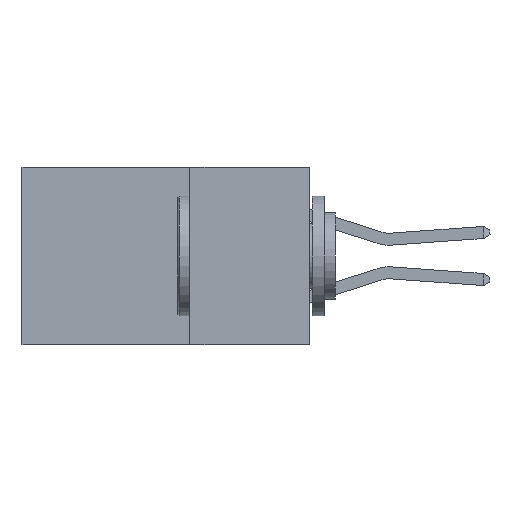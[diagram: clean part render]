
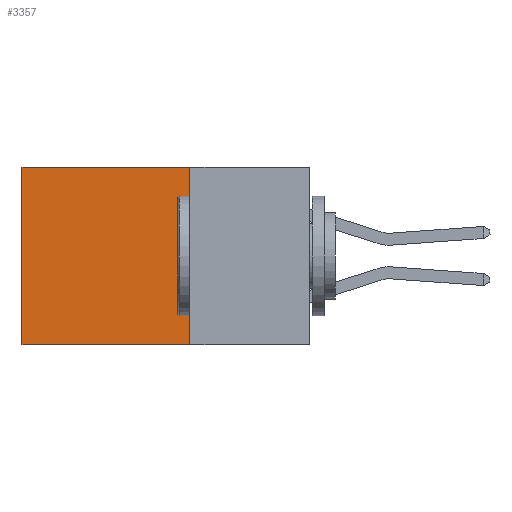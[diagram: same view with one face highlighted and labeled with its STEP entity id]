
A CAD part, left-side view. The second image highlights one B-rep face of the part: STEP entity #3357.
In plain terms, the highlighted planar face has unit normal (-1, 0, 0).
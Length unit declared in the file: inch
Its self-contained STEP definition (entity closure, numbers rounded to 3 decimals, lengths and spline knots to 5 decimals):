
#457 = CARTESIAN_POINT ( 'NONE',  ( 0.298, 0.6, 0. ) ) ;
#503 = CARTESIAN_POINT ( 'NONE',  ( 0.298, 0.25, 0. ) ) ;
#523 = DIRECTION ( 'NONE',  ( 0., 0., -1. ) ) ;
#626 = VECTOR ( 'NONE', #11595, 39.37008 ) ;
#689 = DIRECTION ( 'NONE',  ( 1., 0., 0. ) ) ;
#766 = DIRECTION ( 'NONE',  ( 0., 1., 0. ) ) ;
#1103 = FACE_OUTER_BOUND ( 'NONE', #9966, .T. ) ;
#1236 = LINE ( 'NONE', #457, #626 ) ;
#1303 = CARTESIAN_POINT ( 'NONE',  ( 0.298, 0.25, 0. ) ) ;
#1357 = VECTOR ( 'NONE', #10950, 39.37008 ) ;
#1670 = VERTEX_POINT ( 'NONE', #6899 ) ;
#2214 = ORIENTED_EDGE ( 'NONE', *, *, #8538, .F. ) ;
#2827 = ORIENTED_EDGE ( 'NONE', *, *, #9487, .T. ) ;
#2986 = LINE ( 'NONE', #10077, #10328 ) ;
#3042 = PLANE ( 'NONE',  #4304 ) ;
#3357 = ADVANCED_FACE ( 'NONE', ( #1103 ), #3042, .F. ) ;
#3380 = CARTESIAN_POINT ( 'NONE',  ( 0.298, 0.25, 0. ) ) ;
#4304 = AXIS2_PLACEMENT_3D ( 'NONE', #3380, #689, #523 ) ;
#4399 = CARTESIAN_POINT ( 'NONE',  ( 0.298, 0.6, -0.37 ) ) ;
#5086 = VERTEX_POINT ( 'NONE', #4399 ) ;
#5456 = VERTEX_POINT ( 'NONE', #503 ) ;
#5722 = LINE ( 'NONE', #8233, #1357 ) ;
#5822 = ORIENTED_EDGE ( 'NONE', *, *, #10580, .F. ) ;
#6776 = VECTOR ( 'NONE', #7838, 39.37008 ) ;
#6899 = CARTESIAN_POINT ( 'NONE',  ( 0.298, 0.6, 0. ) ) ;
#7838 = DIRECTION ( 'NONE',  ( 0., 0., -1. ) ) ;
#8233 = CARTESIAN_POINT ( 'NONE',  ( 0.298, 0.25, -0.37 ) ) ;
#8538 = EDGE_CURVE ( 'NONE', #5456, #11982, #8930, .T. ) ;
#8629 = EDGE_CURVE ( 'NONE', #1670, #5086, #1236, .T. ) ;
#8930 = LINE ( 'NONE', #1303, #6776 ) ;
#9487 = EDGE_CURVE ( 'NONE', #5456, #1670, #2986, .T. ) ;
#9966 = EDGE_LOOP ( 'NONE', ( #11088, #5822, #2214, #2827 ) ) ;
#10077 = CARTESIAN_POINT ( 'NONE',  ( 0.298, 0.25, 0. ) ) ;
#10328 = VECTOR ( 'NONE', #766, 39.37008 ) ;
#10580 = EDGE_CURVE ( 'NONE', #11982, #5086, #5722, .T. ) ;
#10950 = DIRECTION ( 'NONE',  ( 0., 1., 0. ) ) ;
#11088 = ORIENTED_EDGE ( 'NONE', *, *, #8629, .T. ) ;
#11595 = DIRECTION ( 'NONE',  ( 0., 0., -1. ) ) ;
#11903 = CARTESIAN_POINT ( 'NONE',  ( 0.298, 0.25, -0.37 ) ) ;
#11982 = VERTEX_POINT ( 'NONE', #11903 ) ;
